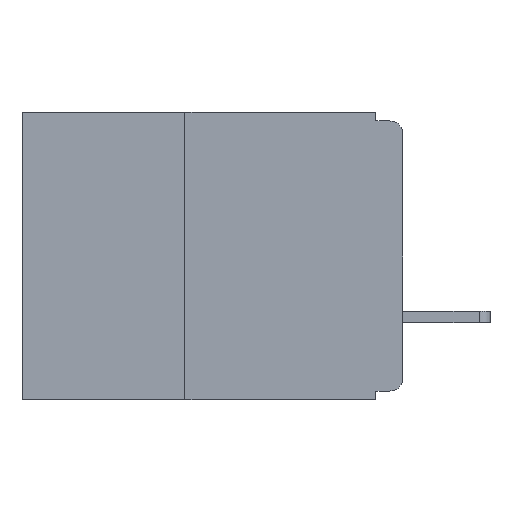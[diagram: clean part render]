
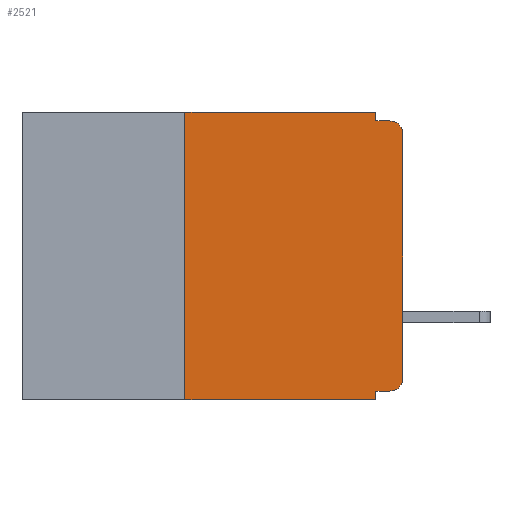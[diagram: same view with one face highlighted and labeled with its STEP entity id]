
A CAD part, left-side view. The second image highlights one B-rep face of the part: STEP entity #2521.
In plain terms, the highlighted planar face has unit normal (-1, 0, 0).
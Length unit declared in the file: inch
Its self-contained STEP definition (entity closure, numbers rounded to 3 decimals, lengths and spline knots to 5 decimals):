
#132 = AXIS2_PLACEMENT_3D ( 'NONE', #13630, #7661, #757 ) ;
#239 = LINE ( 'NONE', #10242, #9047 ) ;
#356 = VERTEX_POINT ( 'NONE', #6002 ) ;
#479 = EDGE_CURVE ( 'NONE', #5014, #1537, #844, .T. ) ;
#757 = DIRECTION ( 'NONE',  ( 0., 0., -1. ) ) ;
#781 = FACE_OUTER_BOUND ( 'NONE', #6427, .T. ) ;
#844 = LINE ( 'NONE', #6082, #3622 ) ;
#988 = VERTEX_POINT ( 'NONE', #11845 ) ;
#1013 = VERTEX_POINT ( 'NONE', #10640 ) ;
#1079 = VECTOR ( 'NONE', #11062, 39.37008 ) ;
#1237 = EDGE_CURVE ( 'NONE', #1537, #10256, #239, .T. ) ;
#1537 = VERTEX_POINT ( 'NONE', #7696 ) ;
#1950 = AXIS2_PLACEMENT_3D ( 'NONE', #10832, #12625, #13817 ) ;
#2521 = ADVANCED_FACE ( 'NONE', ( #781 ), #8281, .F. ) ;
#2524 = DIRECTION ( 'NONE',  ( 0., -1., 0. ) ) ;
#2709 = VECTOR ( 'NONE', #12680, 39.37008 ) ;
#2969 = ORIENTED_EDGE ( 'NONE', *, *, #479, .F. ) ;
#3118 = VECTOR ( 'NONE', #8105, 39.37008 ) ;
#3337 = ORIENTED_EDGE ( 'NONE', *, *, #12815, .T. ) ;
#3622 = VECTOR ( 'NONE', #13802, 39.37008 ) ;
#4179 = LINE ( 'NONE', #4561, #1079 ) ;
#4303 = DIRECTION ( 'NONE',  ( 0., 0., -1. ) ) ;
#4561 = CARTESIAN_POINT ( 'NONE',  ( 0., 0., -0.01 ) ) ;
#4719 = LINE ( 'NONE', #9279, #10506 ) ;
#5014 = VERTEX_POINT ( 'NONE', #10239 ) ;
#5165 = VERTEX_POINT ( 'NONE', #9038 ) ;
#5307 = ORIENTED_EDGE ( 'NONE', *, *, #10859, .T. ) ;
#5469 = CARTESIAN_POINT ( 'NONE',  ( 0., 0.031, -0.33 ) ) ;
#5639 = CIRCLE ( 'NONE', #132, 0.015 ) ;
#5678 = ORIENTED_EDGE ( 'NONE', *, *, #12888, .T. ) ;
#5931 = CARTESIAN_POINT ( 'NONE',  ( 0., 0.015, -0.32 ) ) ;
#6002 = CARTESIAN_POINT ( 'NONE',  ( 0., 0.031, -0.32 ) ) ;
#6082 = CARTESIAN_POINT ( 'NONE',  ( 0., 0.437, 0. ) ) ;
#6138 = LINE ( 'NONE', #8713, #2709 ) ;
#6166 = DIRECTION ( 'NONE',  ( -1., 0., 0. ) ) ;
#6365 = ORIENTED_EDGE ( 'NONE', *, *, #11416, .F. ) ;
#6427 = EDGE_LOOP ( 'NONE', ( #5307, #5678, #8616, #13793, #2969, #8946, #3337, #6365, #9290, #11886 ) ) ;
#6558 = CARTESIAN_POINT ( 'NONE',  ( 0., 0.031, -0.01 ) ) ;
#6659 = CIRCLE ( 'NONE', #13024, 0.015 ) ;
#6669 = LINE ( 'NONE', #9490, #9564 ) ;
#7029 = VECTOR ( 'NONE', #13401, 39.37008 ) ;
#7367 = LINE ( 'NONE', #12439, #7029 ) ;
#7661 = DIRECTION ( 'NONE',  ( -1., 0., 0. ) ) ;
#7696 = CARTESIAN_POINT ( 'NONE',  ( 0., 0.031, 0. ) ) ;
#8105 = DIRECTION ( 'NONE',  ( 0., 0., 1. ) ) ;
#8281 = PLANE ( 'NONE',  #1950 ) ;
#8460 = VERTEX_POINT ( 'NONE', #5931 ) ;
#8616 = ORIENTED_EDGE ( 'NONE', *, *, #11069, .F. ) ;
#8713 = CARTESIAN_POINT ( 'NONE',  ( 0., 0., 0. ) ) ;
#8849 = VERTEX_POINT ( 'NONE', #5469 ) ;
#8946 = ORIENTED_EDGE ( 'NONE', *, *, #11170, .F. ) ;
#9038 = CARTESIAN_POINT ( 'NONE',  ( 0., 0.015, -0.01 ) ) ;
#9047 = VECTOR ( 'NONE', #4303, 39.37008 ) ;
#9089 = LINE ( 'NONE', #13060, #3118 ) ;
#9279 = CARTESIAN_POINT ( 'NONE',  ( 0., 0.437, -0.33 ) ) ;
#9290 = ORIENTED_EDGE ( 'NONE', *, *, #12291, .F. ) ;
#9490 = CARTESIAN_POINT ( 'NONE',  ( 0., 0.031, -0.33 ) ) ;
#9564 = VECTOR ( 'NONE', #10504, 39.37008 ) ;
#10239 = CARTESIAN_POINT ( 'NONE',  ( 0., 0.25, 0. ) ) ;
#10242 = CARTESIAN_POINT ( 'NONE',  ( 0., 0.031, 0. ) ) ;
#10256 = VERTEX_POINT ( 'NONE', #6558 ) ;
#10504 = DIRECTION ( 'NONE',  ( 0., 0., -1. ) ) ;
#10506 = VECTOR ( 'NONE', #2524, 39.37008 ) ;
#10640 = CARTESIAN_POINT ( 'NONE',  ( 0., 0.25, -0.33 ) ) ;
#10721 = VERTEX_POINT ( 'NONE', #13433 ) ;
#10832 = CARTESIAN_POINT ( 'NONE',  ( 0., 0.437, 0. ) ) ;
#10859 = EDGE_CURVE ( 'NONE', #988, #10721, #6138, .T. ) ;
#11062 = DIRECTION ( 'NONE',  ( 0., -1., 0. ) ) ;
#11069 = EDGE_CURVE ( 'NONE', #10256, #5165, #4179, .T. ) ;
#11170 = EDGE_CURVE ( 'NONE', #1013, #5014, #9089, .T. ) ;
#11416 = EDGE_CURVE ( 'NONE', #356, #8849, #6669, .T. ) ;
#11845 = CARTESIAN_POINT ( 'NONE',  ( 0., 0., -0.305 ) ) ;
#11886 = ORIENTED_EDGE ( 'NONE', *, *, #12501, .T. ) ;
#12291 = EDGE_CURVE ( 'NONE', #8460, #356, #7367, .T. ) ;
#12348 = CARTESIAN_POINT ( 'NONE',  ( 0., 0.015, -0.025 ) ) ;
#12439 = CARTESIAN_POINT ( 'NONE',  ( 0., 0., -0.32 ) ) ;
#12501 = EDGE_CURVE ( 'NONE', #8460, #988, #5639, .T. ) ;
#12625 = DIRECTION ( 'NONE',  ( 1., 0., 0. ) ) ;
#12680 = DIRECTION ( 'NONE',  ( 0., 0., 1. ) ) ;
#12815 = EDGE_CURVE ( 'NONE', #1013, #8849, #4719, .T. ) ;
#12888 = EDGE_CURVE ( 'NONE', #10721, #5165, #6659, .T. ) ;
#13024 = AXIS2_PLACEMENT_3D ( 'NONE', #12348, #6166, #13306 ) ;
#13060 = CARTESIAN_POINT ( 'NONE',  ( 0., 0.25, -0.33 ) ) ;
#13306 = DIRECTION ( 'NONE',  ( 0., 0., -1. ) ) ;
#13401 = DIRECTION ( 'NONE',  ( 0., 1., 0. ) ) ;
#13433 = CARTESIAN_POINT ( 'NONE',  ( 0., 0., -0.025 ) ) ;
#13630 = CARTESIAN_POINT ( 'NONE',  ( 0., 0.015, -0.305 ) ) ;
#13793 = ORIENTED_EDGE ( 'NONE', *, *, #1237, .F. ) ;
#13802 = DIRECTION ( 'NONE',  ( 0., -1., 0. ) ) ;
#13817 = DIRECTION ( 'NONE',  ( 0., 0., -1. ) ) ;
